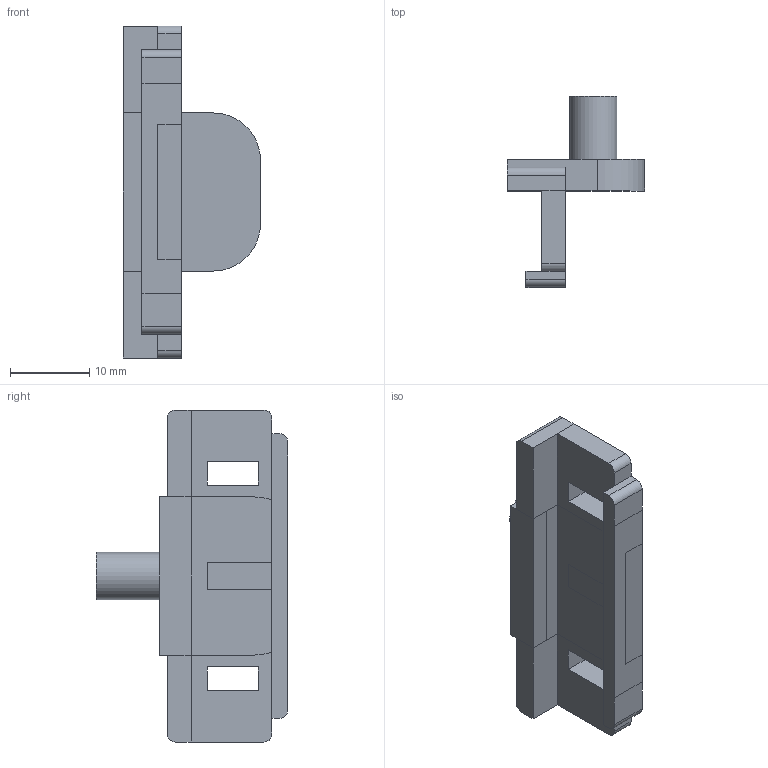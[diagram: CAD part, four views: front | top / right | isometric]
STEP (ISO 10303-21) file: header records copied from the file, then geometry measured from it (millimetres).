
FILE_DESCRIPTION(('FreeCAD Model'),'2;1');
FILE_NAME('ap9 ejector pivot final solution.step','2018-04-08T21:43:59',('Author'),(''), 'Open CASCADE STEP processor 6.8','FreeCAD','Unknown');
FILE_SCHEMA(('AUTOMOTIVE_DESIGN_CC2 { 1 2 10303 214 -1 1 5 4 }'));
Length unit declared in the file: millimetre
Products named in the file (1): Fillet004
Bounding box: 17.34 x 24.2 x 42 mm (x, y, z)
Volume: 3558 mm3; surface area: 2793 mm2
Topology: 1 solids, 1 shells, 60 faces, 159 edges, 102 vertices
Faces by surface type: plane 51, cylinder 9
Full cylindrical faces by diameter (mm): 6 x1
Entity records: 3918 total; most frequent: CARTESIAN_POINT 766, DIRECTION 562, LINE 375, VECTOR 375, ORIENTED_EDGE 318, PCURVE 318, DEFINITIONAL_REPRESENTATION 318, EDGE_CURVE 159
